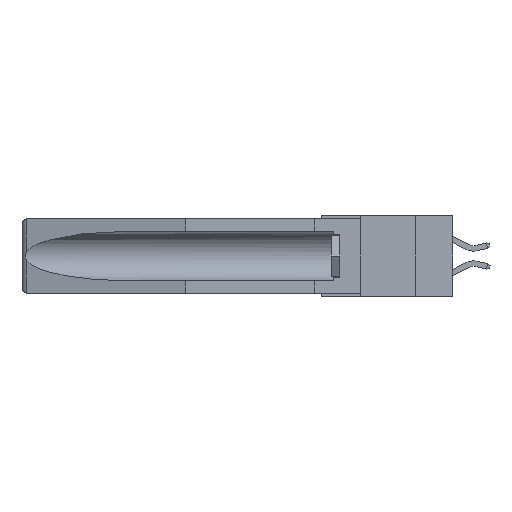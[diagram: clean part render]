
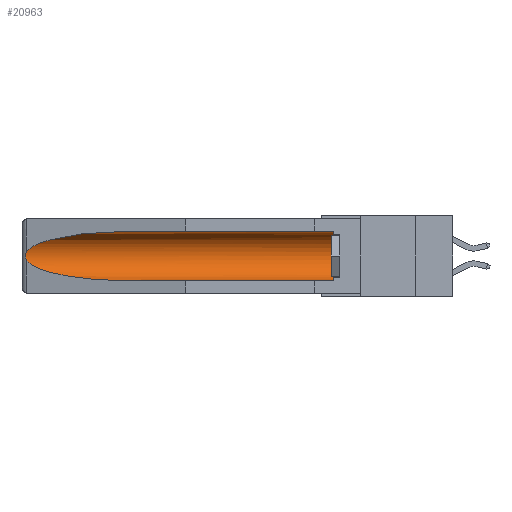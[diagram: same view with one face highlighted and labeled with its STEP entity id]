
A CAD part, left-side view. The second image highlights one B-rep face of the part: STEP entity #20963.
In plain terms, the highlighted cylindrical face has radius 2.857 mm (diameter 5.715 mm), a partial arc.
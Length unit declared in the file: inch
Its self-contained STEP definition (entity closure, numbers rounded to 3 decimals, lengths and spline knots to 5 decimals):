
#174 = CARTESIAN_POINT ( 'NONE',  ( 0.21114, 1.30732, -0.059 ) ) ;
#360 = EDGE_CURVE ( 'NONE', #11624, #19107, #4068, .T. ) ;
#997 = AXIS2_PLACEMENT_3D ( 'NONE', #2946, #19810, #14777 ) ;
#1219 = DIRECTION ( 'NONE',  ( 0., -1., 0. ) ) ;
#1655 =( BOUNDED_CURVE ( )  B_SPLINE_CURVE ( 3, ( #7155, #174, #7001, #3641 ),
 .UNSPECIFIED., .F., .T. ) 
 B_SPLINE_CURVE_WITH_KNOTS ( ( 4, 4 ),
 ( 4.71239, 6.08839 ),
 .UNSPECIFIED. ) 
 CURVE ( )  GEOMETRIC_REPRESENTATION_ITEM ( )  RATIONAL_B_SPLINE_CURVE ( ( 1., 0.848, 0.848, 1. ) ) 
 REPRESENTATION_ITEM ( '' )  );
#1722 = ORIENTED_EDGE ( 'NONE', *, *, #16286, .T. ) ;
#2011 = CARTESIAN_POINT ( 'NONE',  ( 0.155, -0.30754, -0.284 ) ) ;
#2260 = ORIENTED_EDGE ( 'NONE', *, *, #4000, .T. ) ;
#2459 = EDGE_CURVE ( 'NONE', #19107, #16973, #1655, .T. ) ;
#2946 = CARTESIAN_POINT ( 'NONE',  ( 0.155, -0.30754, -0.1715 ) ) ;
#3500 = CARTESIAN_POINT ( 'NONE',  ( 0.155, 1.07973, -0.284 ) ) ;
#3641 = CARTESIAN_POINT ( 'NONE',  ( 0.26537, 1.52718, -0.14972 ) ) ;
#3800 = CARTESIAN_POINT ( 'NONE',  ( 0.26537, 1.52718, -0.19328 ) ) ;
#4000 = EDGE_CURVE ( 'NONE', #20395, #11624, #17486, .T. ) ;
#4068 = LINE ( 'NONE', #14268, #20407 ) ;
#4476 = CARTESIAN_POINT ( 'NONE',  ( 0.26597, 1.5296, -0.19026 ) ) ;
#5027 = B_SPLINE_CURVE_WITH_KNOTS ( 'NONE', 3,
 ( #16324, #7936, #11021, #9481, #19739, #21283, #11157, #14416, #4476, #11323 ),
 .UNSPECIFIED., .F., .F.,
 ( 4, 2, 2, 2, 4 ),
 ( 0., 0.00029, 0.00058, 0.00087, 0.00117 ),
 .UNSPECIFIED. ) ;
#5650 = EDGE_CURVE ( 'NONE', #20395, #21532, #16767, .T. ) ;
#6459 = CYLINDRICAL_SURFACE ( 'NONE', #997, 0.1125 ) ;
#6561 = VERTEX_POINT ( 'NONE', #3800 ) ;
#6698 = ORIENTED_EDGE ( 'NONE', *, *, #5650, .F. ) ;
#7001 = CARTESIAN_POINT ( 'NONE',  ( 0.25451, 1.48313, -0.09465 ) ) ;
#7155 = CARTESIAN_POINT ( 'NONE',  ( 0.155, 1.07973, -0.059 ) ) ;
#7936 = CARTESIAN_POINT ( 'NONE',  ( 0.26597, 1.52961, -0.15275 ) ) ;
#7960 =( BOUNDED_CURVE ( )  B_SPLINE_CURVE ( 3, ( #15106, #11878, #8491, #16902 ),
 .UNSPECIFIED., .F., .T. ) 
 B_SPLINE_CURVE_WITH_KNOTS ( ( 4, 4 ),
 ( 0.1948, 1.5708 ),
 .UNSPECIFIED. ) 
 CURVE ( )  GEOMETRIC_REPRESENTATION_ITEM ( )  RATIONAL_B_SPLINE_CURVE ( ( 1., 0.848, 0.848, 1. ) ) 
 REPRESENTATION_ITEM ( '' )  );
#8491 = CARTESIAN_POINT ( 'NONE',  ( 0.21114, 1.30732, -0.284 ) ) ;
#9099 = DIRECTION ( 'NONE',  ( 0., 1., 0. ) ) ;
#9206 = AXIS2_PLACEMENT_3D ( 'NONE', #11304, #1219, #14686 ) ;
#9275 = ORIENTED_EDGE ( 'NONE', *, *, #2459, .T. ) ;
#9481 = CARTESIAN_POINT ( 'NONE',  ( 0.2673, 1.5327, -0.16383 ) ) ;
#10410 = CARTESIAN_POINT ( 'NONE',  ( 0.155, 0.126, -0.059 ) ) ;
#11021 = CARTESIAN_POINT ( 'NONE',  ( 0.26654, 1.53092, -0.15636 ) ) ;
#11157 = CARTESIAN_POINT ( 'NONE',  ( 0.2673, 1.53269, -0.17917 ) ) ;
#11202 = ORIENTED_EDGE ( 'NONE', *, *, #360, .T. ) ;
#11304 = CARTESIAN_POINT ( 'NONE',  ( 0.155, 0.126, -0.1715 ) ) ;
#11323 = CARTESIAN_POINT ( 'NONE',  ( 0.26537, 1.52718, -0.19328 ) ) ;
#11624 = VERTEX_POINT ( 'NONE', #10410 ) ;
#11741 = VECTOR ( 'NONE', #17030, 39.37008 ) ;
#11878 = CARTESIAN_POINT ( 'NONE',  ( 0.25451, 1.48313, -0.24835 ) ) ;
#12783 = CARTESIAN_POINT ( 'NONE',  ( 0.155, 1.07973, -0.059 ) ) ;
#14002 = ORIENTED_EDGE ( 'NONE', *, *, #18279, .T. ) ;
#14268 = CARTESIAN_POINT ( 'NONE',  ( 0.155, -0.30754, -0.059 ) ) ;
#14416 = CARTESIAN_POINT ( 'NONE',  ( 0.26655, 1.53094, -0.18657 ) ) ;
#14686 = DIRECTION ( 'NONE',  ( 0., 0., 1. ) ) ;
#14777 = DIRECTION ( 'NONE',  ( 0., 0., 1. ) ) ;
#15106 = CARTESIAN_POINT ( 'NONE',  ( 0.26537, 1.52718, -0.19328 ) ) ;
#16286 = EDGE_CURVE ( 'NONE', #6561, #21532, #7960, .T. ) ;
#16324 = CARTESIAN_POINT ( 'NONE',  ( 0.26537, 1.52718, -0.14972 ) ) ;
#16767 = LINE ( 'NONE', #2011, #11741 ) ;
#16902 = CARTESIAN_POINT ( 'NONE',  ( 0.155, 1.07973, -0.284 ) ) ;
#16973 = VERTEX_POINT ( 'NONE', #17881 ) ;
#17030 = DIRECTION ( 'NONE',  ( 0., 1., 0. ) ) ;
#17061 = FACE_OUTER_BOUND ( 'NONE', #21279, .T. ) ;
#17486 = CIRCLE ( 'NONE', #9206, 0.1125 ) ;
#17881 = CARTESIAN_POINT ( 'NONE',  ( 0.26537, 1.52718, -0.14972 ) ) ;
#18011 = CARTESIAN_POINT ( 'NONE',  ( 0.155, 0.126, -0.284 ) ) ;
#18279 = EDGE_CURVE ( 'NONE', #16973, #6561, #5027, .T. ) ;
#19107 = VERTEX_POINT ( 'NONE', #12783 ) ;
#19739 = CARTESIAN_POINT ( 'NONE',  ( 0.2675, 1.53308, -0.16763 ) ) ;
#19810 = DIRECTION ( 'NONE',  ( 0., 1., 0. ) ) ;
#20395 = VERTEX_POINT ( 'NONE', #18011 ) ;
#20407 = VECTOR ( 'NONE', #9099, 39.37008 ) ;
#20963 = ADVANCED_FACE ( 'NONE', ( #17061 ), #6459, .F. ) ;
#21279 = EDGE_LOOP ( 'NONE', ( #9275, #14002, #1722, #6698, #2260, #11202 ) ) ;
#21283 = CARTESIAN_POINT ( 'NONE',  ( 0.2675, 1.53308, -0.17534 ) ) ;
#21532 = VERTEX_POINT ( 'NONE', #3500 ) ;
